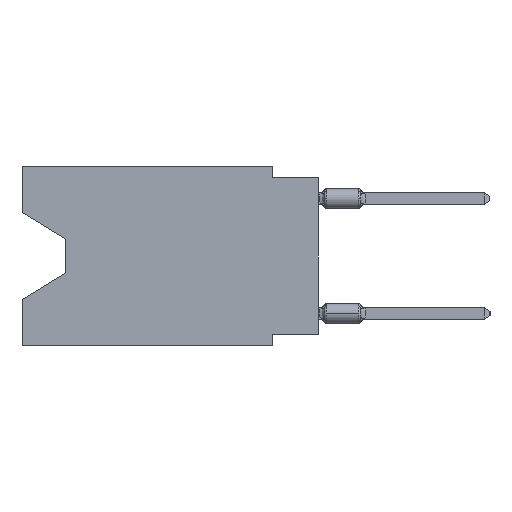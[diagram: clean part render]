
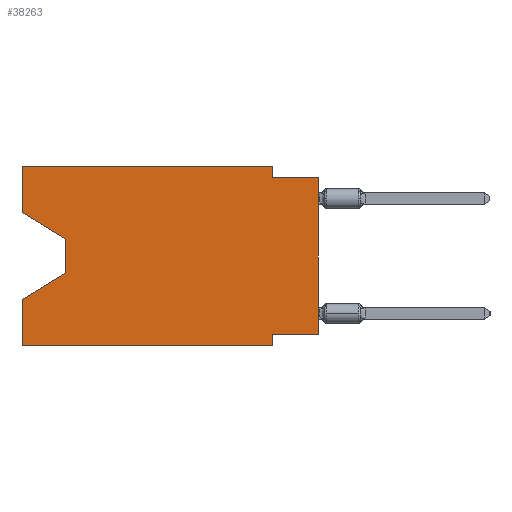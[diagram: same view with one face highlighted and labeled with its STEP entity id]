
A CAD part, left-side view. The second image highlights one B-rep face of the part: STEP entity #38263.
In plain terms, the highlighted planar face has unit normal (-1, 0, 0).
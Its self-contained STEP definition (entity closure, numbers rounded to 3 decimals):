
#4 = DIRECTION ( 'NONE',  ( 0., -0.855, -0.519 ) ) ;
#221 = CARTESIAN_POINT ( 'NONE',  ( 0., 16.383, 0. ) ) ;
#305 = EDGE_CURVE ( 'NONE', #6708, #30171, #23813, .T. ) ;
#544 = CARTESIAN_POINT ( 'NONE',  ( 0., 2.54, 0. ) ) ;
#1027 = ORIENTED_EDGE ( 'NONE', *, *, #23339, .F. ) ;
#1500 = AXIS2_PLACEMENT_3D ( 'NONE', #26337, #23536, #5087 ) ;
#2397 = CARTESIAN_POINT ( 'NONE',  ( 0., 16.383, -7.36 ) ) ;
#2443 = VECTOR ( 'NONE', #27842, 1000. ) ;
#2789 = VERTEX_POINT ( 'NONE', #25903 ) ;
#2957 = DIRECTION ( 'NONE',  ( 0., -1., 0. ) ) ;
#3142 = CARTESIAN_POINT ( 'NONE',  ( 0., 2.54, -0.635 ) ) ;
#3307 = CARTESIAN_POINT ( 'NONE',  ( 0., 16.383, 0. ) ) ;
#4696 = CARTESIAN_POINT ( 'NONE',  ( 0., 13.97, -4.013 ) ) ;
#5012 = EDGE_CURVE ( 'NONE', #36090, #33665, #27636, .T. ) ;
#5087 = DIRECTION ( 'NONE',  ( 0., 0., -1. ) ) ;
#5464 = DIRECTION ( 'NONE',  ( 0., -1., 0. ) ) ;
#5659 = CARTESIAN_POINT ( 'NONE',  ( 0., 13.97, -5.893 ) ) ;
#6303 = ORIENTED_EDGE ( 'NONE', *, *, #30557, .F. ) ;
#6314 = LINE ( 'NONE', #3307, #18208 ) ;
#6386 = CARTESIAN_POINT ( 'NONE',  ( 0., 0., -9.271 ) ) ;
#6460 = VECTOR ( 'NONE', #14992, 1000. ) ;
#6708 = VERTEX_POINT ( 'NONE', #17271 ) ;
#6807 = EDGE_CURVE ( 'NONE', #2789, #38212, #39296, .T. ) ;
#6832 = LINE ( 'NONE', #31275, #27768 ) ;
#7107 = VECTOR ( 'NONE', #4, 1000. ) ;
#7154 = DIRECTION ( 'NONE',  ( 0., 0., -1. ) ) ;
#7676 = EDGE_CURVE ( 'NONE', #14313, #37345, #8323, .T. ) ;
#8323 = LINE ( 'NONE', #30891, #33430 ) ;
#8378 = ORIENTED_EDGE ( 'NONE', *, *, #38990, .F. ) ;
#9234 = CARTESIAN_POINT ( 'NONE',  ( 0., 13.97, -4.013 ) ) ;
#9374 = ORIENTED_EDGE ( 'NONE', *, *, #24415, .F. ) ;
#10414 = VERTEX_POINT ( 'NONE', #544 ) ;
#10809 = LINE ( 'NONE', #23047, #6460 ) ;
#10899 = ORIENTED_EDGE ( 'NONE', *, *, #5012, .F. ) ;
#11184 = DIRECTION ( 'NONE',  ( 0., 0., 1. ) ) ;
#11503 = ORIENTED_EDGE ( 'NONE', *, *, #7676, .T. ) ;
#11675 = DIRECTION ( 'NONE',  ( 0., 0., 1. ) ) ;
#12459 = DIRECTION ( 'NONE',  ( 0., 0.855, -0.519 ) ) ;
#13769 = LINE ( 'NONE', #25618, #25273 ) ;
#13836 = CARTESIAN_POINT ( 'NONE',  ( 0., 2.54, -9.271 ) ) ;
#13864 = VECTOR ( 'NONE', #11675, 1000. ) ;
#14179 = LINE ( 'NONE', #35040, #38911 ) ;
#14313 = VERTEX_POINT ( 'NONE', #5659 ) ;
#14992 = DIRECTION ( 'NONE',  ( 0., -1., 0. ) ) ;
#16103 = CARTESIAN_POINT ( 'NONE',  ( 0., 2.54, -9.906 ) ) ;
#17271 = CARTESIAN_POINT ( 'NONE',  ( 0., 16.383, -9.906 ) ) ;
#17700 = LINE ( 'NONE', #29921, #13864 ) ;
#17940 = VERTEX_POINT ( 'NONE', #221 ) ;
#18208 = VECTOR ( 'NONE', #24763, 1000. ) ;
#18732 = CARTESIAN_POINT ( 'NONE',  ( 0., 0., -9.271 ) ) ;
#18758 = ORIENTED_EDGE ( 'NONE', *, *, #22872, .F. ) ;
#22872 = EDGE_CURVE ( 'NONE', #10414, #27029, #6832, .T. ) ;
#23047 = CARTESIAN_POINT ( 'NONE',  ( 0., 16.383, 0. ) ) ;
#23339 = EDGE_CURVE ( 'NONE', #2789, #17940, #6314, .T. ) ;
#23536 = DIRECTION ( 'NONE',  ( 1., 0., 0. ) ) ;
#23700 = LINE ( 'NONE', #32902, #37628 ) ;
#23813 = LINE ( 'NONE', #24797, #35725 ) ;
#24196 = ORIENTED_EDGE ( 'NONE', *, *, #305, .T. ) ;
#24415 = EDGE_CURVE ( 'NONE', #17940, #10414, #10809, .T. ) ;
#24763 = DIRECTION ( 'NONE',  ( 0., 0., 1. ) ) ;
#24797 = CARTESIAN_POINT ( 'NONE',  ( 0., 16.383, -9.906 ) ) ;
#25273 = VECTOR ( 'NONE', #7154, 1000. ) ;
#25618 = CARTESIAN_POINT ( 'NONE',  ( 0., 2.54, -9.906 ) ) ;
#25903 = CARTESIAN_POINT ( 'NONE',  ( 0., 16.383, -2.546 ) ) ;
#26337 = CARTESIAN_POINT ( 'NONE',  ( 0., 16.383, 0. ) ) ;
#27029 = VERTEX_POINT ( 'NONE', #3142 ) ;
#27272 = EDGE_LOOP ( 'NONE', ( #34168, #33467, #11503, #34326, #24196, #8378, #10899, #30936, #6303, #18758, #9374, #1027 ) ) ;
#27636 = LINE ( 'NONE', #6386, #2443 ) ;
#27768 = VECTOR ( 'NONE', #37295, 1000. ) ;
#27842 = DIRECTION ( 'NONE',  ( 0., 1., 0. ) ) ;
#29431 = EDGE_CURVE ( 'NONE', #38212, #14313, #37092, .T. ) ;
#29921 = CARTESIAN_POINT ( 'NONE',  ( 0., 16.383, 0. ) ) ;
#30171 = VERTEX_POINT ( 'NONE', #16103 ) ;
#30557 = EDGE_CURVE ( 'NONE', #27029, #32990, #23700, .T. ) ;
#30891 = CARTESIAN_POINT ( 'NONE',  ( 0., 13.97, -5.893 ) ) ;
#30936 = ORIENTED_EDGE ( 'NONE', *, *, #30963, .T. ) ;
#30963 = EDGE_CURVE ( 'NONE', #36090, #32990, #14179, .T. ) ;
#31125 = CARTESIAN_POINT ( 'NONE',  ( 0., 0., -0.635 ) ) ;
#31275 = CARTESIAN_POINT ( 'NONE',  ( 0., 2.54, 0. ) ) ;
#32335 = PLANE ( 'NONE',  #1500 ) ;
#32537 = FACE_OUTER_BOUND ( 'NONE', #27272, .T. ) ;
#32902 = CARTESIAN_POINT ( 'NONE',  ( 0., 0., -0.635 ) ) ;
#32990 = VERTEX_POINT ( 'NONE', #31125 ) ;
#33430 = VECTOR ( 'NONE', #12459, 1000. ) ;
#33467 = ORIENTED_EDGE ( 'NONE', *, *, #29431, .T. ) ;
#33665 = VERTEX_POINT ( 'NONE', #13836 ) ;
#34168 = ORIENTED_EDGE ( 'NONE', *, *, #6807, .T. ) ;
#34326 = ORIENTED_EDGE ( 'NONE', *, *, #36391, .F. ) ;
#35040 = CARTESIAN_POINT ( 'NONE',  ( 0., 0., 0. ) ) ;
#35725 = VECTOR ( 'NONE', #2957, 1000. ) ;
#36090 = VERTEX_POINT ( 'NONE', #18732 ) ;
#36391 = EDGE_CURVE ( 'NONE', #6708, #37345, #17700, .T. ) ;
#36871 = VECTOR ( 'NONE', #39497, 1000. ) ;
#36883 = CARTESIAN_POINT ( 'NONE',  ( 0., 16.383, -2.546 ) ) ;
#37092 = LINE ( 'NONE', #9234, #36871 ) ;
#37295 = DIRECTION ( 'NONE',  ( 0., 0., -1. ) ) ;
#37345 = VERTEX_POINT ( 'NONE', #2397 ) ;
#37628 = VECTOR ( 'NONE', #5464, 1000. ) ;
#38212 = VERTEX_POINT ( 'NONE', #4696 ) ;
#38263 = ADVANCED_FACE ( 'NONE', ( #32537 ), #32335, .F. ) ;
#38911 = VECTOR ( 'NONE', #11184, 1000. ) ;
#38990 = EDGE_CURVE ( 'NONE', #33665, #30171, #13769, .T. ) ;
#39296 = LINE ( 'NONE', #36883, #7107 ) ;
#39497 = DIRECTION ( 'NONE',  ( 0., 0., -1. ) ) ;
